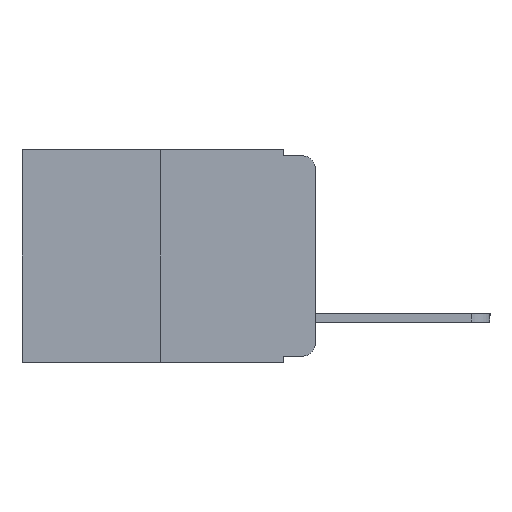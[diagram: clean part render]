
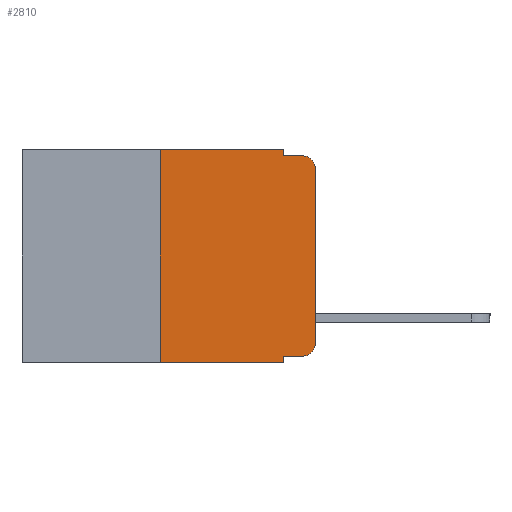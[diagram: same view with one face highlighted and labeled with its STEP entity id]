
A CAD part, left-side view. The second image highlights one B-rep face of the part: STEP entity #2810.
In plain terms, the highlighted planar face has unit normal (-1, 0, 0).
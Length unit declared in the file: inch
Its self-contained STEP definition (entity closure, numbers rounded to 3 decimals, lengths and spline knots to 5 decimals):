
#218 = VERTEX_POINT ( 'NONE', #1111 ) ;
#406 = DIRECTION ( 'NONE',  ( 0., 0., 1. ) ) ;
#783 = LINE ( 'NONE', #3503, #10967 ) ;
#828 = LINE ( 'NONE', #10488, #10615 ) ;
#1111 = CARTESIAN_POINT ( 'NONE',  ( 0., 0.051, -0.01 ) ) ;
#1456 = VERTEX_POINT ( 'NONE', #9669 ) ;
#1772 = CARTESIAN_POINT ( 'NONE',  ( 0., 0.02, -0.313 ) ) ;
#1846 = CARTESIAN_POINT ( 'NONE',  ( 0., 0., -0.03 ) ) ;
#1877 = ORIENTED_EDGE ( 'NONE', *, *, #16398, .T. ) ;
#2025 = CARTESIAN_POINT ( 'NONE',  ( 0., 0., 0. ) ) ;
#2037 = EDGE_LOOP ( 'NONE', ( #13512, #4286, #13895, #4672, #5076, #8285, #11435, #14669, #1877, #8665 ) ) ;
#2075 = EDGE_CURVE ( 'NONE', #1456, #8402, #783, .T. ) ;
#2638 = CARTESIAN_POINT ( 'NONE',  ( 0., 0.051, 0. ) ) ;
#2810 = ADVANCED_FACE ( 'NONE', ( #6523 ), #10848, .F. ) ;
#3201 = DIRECTION ( 'NONE',  ( 0., 0., -1. ) ) ;
#3503 = CARTESIAN_POINT ( 'NONE',  ( 0., 0.051, 0. ) ) ;
#3515 = VECTOR ( 'NONE', #3979, 39.37008 ) ;
#3544 = DIRECTION ( 'NONE',  ( 0., -1., 0. ) ) ;
#3565 = CARTESIAN_POINT ( 'NONE',  ( 0., 0.051, -0.01 ) ) ;
#3606 = CARTESIAN_POINT ( 'NONE',  ( 0., 0.473, 0. ) ) ;
#3868 = EDGE_CURVE ( 'NONE', #9918, #8402, #15841, .T. ) ;
#3971 = EDGE_CURVE ( 'NONE', #9918, #4002, #5530, .T. ) ;
#3979 = DIRECTION ( 'NONE',  ( 0., -1., 0. ) ) ;
#4002 = VERTEX_POINT ( 'NONE', #8078 ) ;
#4286 = ORIENTED_EDGE ( 'NONE', *, *, #7307, .T. ) ;
#4672 = ORIENTED_EDGE ( 'NONE', *, *, #4814, .F. ) ;
#4814 = EDGE_CURVE ( 'NONE', #12693, #218, #10652, .T. ) ;
#4886 = DIRECTION ( 'NONE',  ( 0., 0., -1. ) ) ;
#5019 = DIRECTION ( 'NONE',  ( 0., 0., 1. ) ) ;
#5076 = ORIENTED_EDGE ( 'NONE', *, *, #6796, .F. ) ;
#5168 = CIRCLE ( 'NONE', #13573, 0.02 ) ;
#5361 = CARTESIAN_POINT ( 'NONE',  ( 0., 0.25, -0.343 ) ) ;
#5530 = LINE ( 'NONE', #6128, #11871 ) ;
#5666 = EDGE_CURVE ( 'NONE', #218, #10700, #14246, .T. ) ;
#5895 = CARTESIAN_POINT ( 'NONE',  ( 0., 0.02, -0.03 ) ) ;
#6128 = CARTESIAN_POINT ( 'NONE',  ( 0., 0.25, 0. ) ) ;
#6333 = VERTEX_POINT ( 'NONE', #9765 ) ;
#6523 = FACE_OUTER_BOUND ( 'NONE', #2037, .T. ) ;
#6796 = EDGE_CURVE ( 'NONE', #4002, #12693, #828, .T. ) ;
#7107 = DIRECTION ( 'NONE',  ( 0., 0., -1. ) ) ;
#7307 = EDGE_CURVE ( 'NONE', #13352, #10700, #10604, .T. ) ;
#7422 = DIRECTION ( 'NONE',  ( 0., 0., -1. ) ) ;
#7492 = DIRECTION ( 'NONE',  ( 0., 0., -1. ) ) ;
#7898 = VECTOR ( 'NONE', #3544, 39.37008 ) ;
#8078 = CARTESIAN_POINT ( 'NONE',  ( 0., 0.25, 0. ) ) ;
#8139 = VERTEX_POINT ( 'NONE', #13426 ) ;
#8285 = ORIENTED_EDGE ( 'NONE', *, *, #3971, .F. ) ;
#8402 = VERTEX_POINT ( 'NONE', #16318 ) ;
#8406 = DIRECTION ( 'NONE',  ( 0., -1., 0. ) ) ;
#8665 = ORIENTED_EDGE ( 'NONE', *, *, #15595, .T. ) ;
#8858 = EDGE_CURVE ( 'NONE', #8139, #13352, #9012, .T. ) ;
#9012 = LINE ( 'NONE', #2025, #15032 ) ;
#9602 = LINE ( 'NONE', #11180, #3515 ) ;
#9669 = CARTESIAN_POINT ( 'NONE',  ( 0., 0.051, -0.333 ) ) ;
#9765 = CARTESIAN_POINT ( 'NONE',  ( 0., 0.02, -0.333 ) ) ;
#9918 = VERTEX_POINT ( 'NONE', #5361 ) ;
#10426 = DIRECTION ( 'NONE',  ( 0., -1., 0. ) ) ;
#10488 = CARTESIAN_POINT ( 'NONE',  ( 0., 0.473, 0. ) ) ;
#10511 = DIRECTION ( 'NONE',  ( -1., 0., 0. ) ) ;
#10594 = CARTESIAN_POINT ( 'NONE',  ( 0., 0.473, -0.343 ) ) ;
#10604 = CIRCLE ( 'NONE', #11540, 0.02 ) ;
#10615 = VECTOR ( 'NONE', #10426, 39.37008 ) ;
#10652 = LINE ( 'NONE', #2638, #15972 ) ;
#10700 = VERTEX_POINT ( 'NONE', #14252 ) ;
#10848 = PLANE ( 'NONE',  #14443 ) ;
#10967 = VECTOR ( 'NONE', #7492, 39.37008 ) ;
#11180 = CARTESIAN_POINT ( 'NONE',  ( 0., 0.051, -0.333 ) ) ;
#11435 = ORIENTED_EDGE ( 'NONE', *, *, #3868, .T. ) ;
#11540 = AXIS2_PLACEMENT_3D ( 'NONE', #5895, #14242, #7107 ) ;
#11789 = CARTESIAN_POINT ( 'NONE',  ( 0., 0.051, 0. ) ) ;
#11871 = VECTOR ( 'NONE', #5019, 39.37008 ) ;
#12089 = DIRECTION ( 'NONE',  ( 1., 0., 0. ) ) ;
#12636 = VECTOR ( 'NONE', #8406, 39.37008 ) ;
#12693 = VERTEX_POINT ( 'NONE', #11789 ) ;
#13352 = VERTEX_POINT ( 'NONE', #1846 ) ;
#13426 = CARTESIAN_POINT ( 'NONE',  ( 0., 0., -0.313 ) ) ;
#13512 = ORIENTED_EDGE ( 'NONE', *, *, #8858, .T. ) ;
#13573 = AXIS2_PLACEMENT_3D ( 'NONE', #1772, #10511, #3201 ) ;
#13895 = ORIENTED_EDGE ( 'NONE', *, *, #5666, .F. ) ;
#14242 = DIRECTION ( 'NONE',  ( -1., 0., 0. ) ) ;
#14246 = LINE ( 'NONE', #3565, #7898 ) ;
#14252 = CARTESIAN_POINT ( 'NONE',  ( 0., 0.02, -0.01 ) ) ;
#14443 = AXIS2_PLACEMENT_3D ( 'NONE', #3606, #12089, #4886 ) ;
#14669 = ORIENTED_EDGE ( 'NONE', *, *, #2075, .F. ) ;
#15032 = VECTOR ( 'NONE', #406, 39.37008 ) ;
#15595 = EDGE_CURVE ( 'NONE', #6333, #8139, #5168, .T. ) ;
#15841 = LINE ( 'NONE', #10594, #12636 ) ;
#15972 = VECTOR ( 'NONE', #7422, 39.37008 ) ;
#16318 = CARTESIAN_POINT ( 'NONE',  ( 0., 0.051, -0.343 ) ) ;
#16398 = EDGE_CURVE ( 'NONE', #1456, #6333, #9602, .T. ) ;
